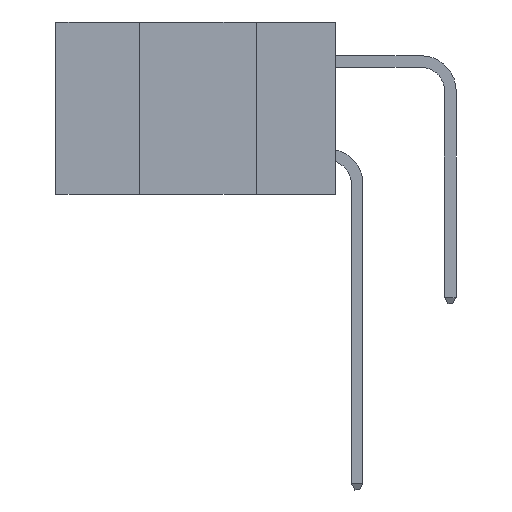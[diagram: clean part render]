
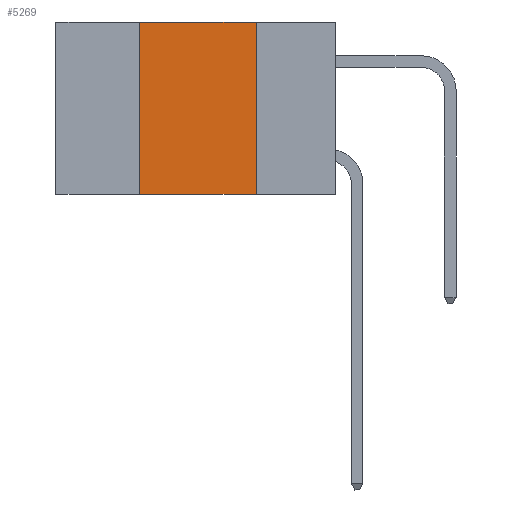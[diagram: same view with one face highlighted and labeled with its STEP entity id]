
A CAD part, left-side view. The second image highlights one B-rep face of the part: STEP entity #5269.
In plain terms, the highlighted planar face has unit normal (-1, 0, 0).
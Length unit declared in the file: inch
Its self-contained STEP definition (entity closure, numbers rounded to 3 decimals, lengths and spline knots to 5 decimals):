
#346 = DIRECTION ( 'NONE',  ( 0., 0., 1. ) ) ;
#657 = DIRECTION ( 'NONE',  ( 1., 0., 0. ) ) ;
#783 = CARTESIAN_POINT ( 'NONE',  ( 0., 0.17, 0. ) ) ;
#792 = EDGE_CURVE ( 'NONE', #4784, #11706, #11309, .T. ) ;
#979 = CARTESIAN_POINT ( 'NONE',  ( 0., 0.17, 0. ) ) ;
#996 = EDGE_CURVE ( 'NONE', #9720, #11706, #6765, .T. ) ;
#1079 = CARTESIAN_POINT ( 'NONE',  ( 0., 0.6, -0.37 ) ) ;
#1382 = LINE ( 'NONE', #3799, #3796 ) ;
#1491 = EDGE_CURVE ( 'NONE', #9720, #9003, #8968, .T. ) ;
#3796 = VECTOR ( 'NONE', #10450, 39.37008 ) ;
#3799 = CARTESIAN_POINT ( 'NONE',  ( 0., 0.6, 0. ) ) ;
#4151 = CARTESIAN_POINT ( 'NONE',  ( 0., 0.42, 0. ) ) ;
#4342 = CARTESIAN_POINT ( 'NONE',  ( 0., 0.42, -0.37 ) ) ;
#4545 = ORIENTED_EDGE ( 'NONE', *, *, #1491, .F. ) ;
#4784 = VERTEX_POINT ( 'NONE', #979 ) ;
#4988 = ORIENTED_EDGE ( 'NONE', *, *, #792, .F. ) ;
#5269 = ADVANCED_FACE ( 'NONE', ( #7241 ), #6645, .F. ) ;
#6357 = CARTESIAN_POINT ( 'NONE',  ( 0., 0.42, 0. ) ) ;
#6462 = VECTOR ( 'NONE', #7456, 39.37008 ) ;
#6645 = PLANE ( 'NONE',  #10516 ) ;
#6765 = LINE ( 'NONE', #1079, #6462 ) ;
#7241 = FACE_OUTER_BOUND ( 'NONE', #8037, .T. ) ;
#7366 = CARTESIAN_POINT ( 'NONE',  ( 0., 0.17, -0.37 ) ) ;
#7456 = DIRECTION ( 'NONE',  ( 0., -1., 0. ) ) ;
#7596 = DIRECTION ( 'NONE',  ( 0., 0., -1. ) ) ;
#8000 = ORIENTED_EDGE ( 'NONE', *, *, #996, .T. ) ;
#8037 = EDGE_LOOP ( 'NONE', ( #4988, #11789, #4545, #8000 ) ) ;
#8968 = LINE ( 'NONE', #6357, #10837 ) ;
#9003 = VERTEX_POINT ( 'NONE', #4151 ) ;
#9720 = VERTEX_POINT ( 'NONE', #4342 ) ;
#10450 = DIRECTION ( 'NONE',  ( 0., -1., 0. ) ) ;
#10516 = AXIS2_PLACEMENT_3D ( 'NONE', #11319, #657, #7596 ) ;
#10837 = VECTOR ( 'NONE', #346, 39.37008 ) ;
#11009 = VECTOR ( 'NONE', #12456, 39.37008 ) ;
#11139 = EDGE_CURVE ( 'NONE', #9003, #4784, #1382, .T. ) ;
#11309 = LINE ( 'NONE', #783, #11009 ) ;
#11319 = CARTESIAN_POINT ( 'NONE',  ( 0., 0.6, 0. ) ) ;
#11706 = VERTEX_POINT ( 'NONE', #7366 ) ;
#11789 = ORIENTED_EDGE ( 'NONE', *, *, #11139, .F. ) ;
#12456 = DIRECTION ( 'NONE',  ( 0., 0., -1. ) ) ;
